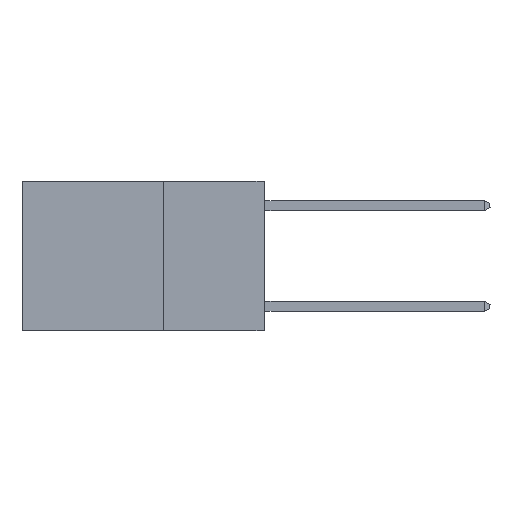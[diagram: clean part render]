
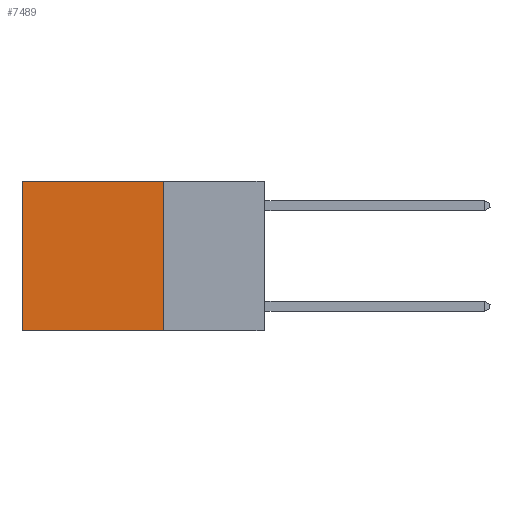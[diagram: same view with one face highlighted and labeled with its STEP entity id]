
A CAD part, left-side view. The second image highlights one B-rep face of the part: STEP entity #7489.
In plain terms, the highlighted planar face has unit normal (-1, 0, 0).
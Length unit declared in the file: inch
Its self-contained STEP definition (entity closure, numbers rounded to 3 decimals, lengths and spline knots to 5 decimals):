
#851 = CARTESIAN_POINT ( 'NONE',  ( 0.2625, 0.25, 0. ) ) ;
#889 = EDGE_LOOP ( 'NONE', ( #27093, #15359, #20093, #30856 ) ) ;
#1233 = LINE ( 'NONE', #7847, #26673 ) ;
#1997 = LINE ( 'NONE', #26763, #14772 ) ;
#2863 = VERTEX_POINT ( 'NONE', #12317 ) ;
#5000 = CARTESIAN_POINT ( 'NONE',  ( 0.2625, 0.6, 0. ) ) ;
#7360 = AXIS2_PLACEMENT_3D ( 'NONE', #23424, #10901, #28488 ) ;
#7489 = ADVANCED_FACE ( 'NONE', ( #30365 ), #8379, .F. ) ;
#7781 = LINE ( 'NONE', #30252, #26285 ) ;
#7847 = CARTESIAN_POINT ( 'NONE',  ( 0.2625, 0.25, -0.37 ) ) ;
#8379 = PLANE ( 'NONE',  #7360 ) ;
#8575 = EDGE_CURVE ( 'NONE', #10945, #23876, #12588, .T. ) ;
#10353 = DIRECTION ( 'NONE',  ( 0., 1., 0. ) ) ;
#10901 = DIRECTION ( 'NONE',  ( 1., 0., 0. ) ) ;
#10945 = VERTEX_POINT ( 'NONE', #5000 ) ;
#10983 = EDGE_CURVE ( 'NONE', #2863, #23876, #1233, .T. ) ;
#11368 = EDGE_CURVE ( 'NONE', #11891, #2863, #1997, .T. ) ;
#11891 = VERTEX_POINT ( 'NONE', #851 ) ;
#12317 = CARTESIAN_POINT ( 'NONE',  ( 0.2625, 0.25, -0.37 ) ) ;
#12588 = LINE ( 'NONE', #15100, #19276 ) ;
#14772 = VECTOR ( 'NONE', #29245, 39.37008 ) ;
#15100 = CARTESIAN_POINT ( 'NONE',  ( 0.2625, 0.6, 0. ) ) ;
#15359 = ORIENTED_EDGE ( 'NONE', *, *, #10983, .F. ) ;
#19276 = VECTOR ( 'NONE', #32681, 39.37008 ) ;
#19765 = EDGE_CURVE ( 'NONE', #11891, #10945, #7781, .T. ) ;
#20093 = ORIENTED_EDGE ( 'NONE', *, *, #11368, .F. ) ;
#20737 = CARTESIAN_POINT ( 'NONE',  ( 0.2625, 0.6, -0.37 ) ) ;
#23424 = CARTESIAN_POINT ( 'NONE',  ( 0.2625, 0.25, 0. ) ) ;
#23876 = VERTEX_POINT ( 'NONE', #20737 ) ;
#26285 = VECTOR ( 'NONE', #32782, 39.37008 ) ;
#26673 = VECTOR ( 'NONE', #10353, 39.37008 ) ;
#26763 = CARTESIAN_POINT ( 'NONE',  ( 0.2625, 0.25, 0. ) ) ;
#27093 = ORIENTED_EDGE ( 'NONE', *, *, #8575, .T. ) ;
#28488 = DIRECTION ( 'NONE',  ( 0., 0., -1. ) ) ;
#29245 = DIRECTION ( 'NONE',  ( 0., 0., -1. ) ) ;
#30252 = CARTESIAN_POINT ( 'NONE',  ( 0.2625, 0.25, 0. ) ) ;
#30365 = FACE_OUTER_BOUND ( 'NONE', #889, .T. ) ;
#30856 = ORIENTED_EDGE ( 'NONE', *, *, #19765, .T. ) ;
#32681 = DIRECTION ( 'NONE',  ( 0., 0., -1. ) ) ;
#32782 = DIRECTION ( 'NONE',  ( 0., 1., 0. ) ) ;
